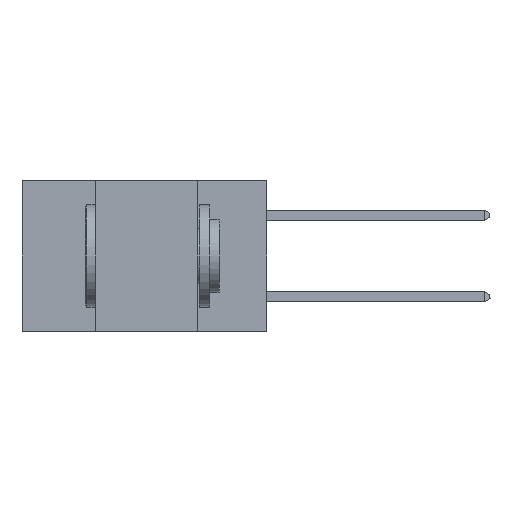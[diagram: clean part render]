
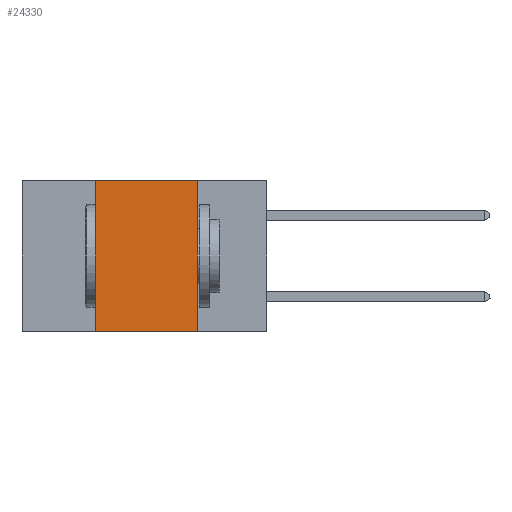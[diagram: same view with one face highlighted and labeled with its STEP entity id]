
A CAD part, left-side view. The second image highlights one B-rep face of the part: STEP entity #24330.
In plain terms, the highlighted planar face has unit normal (-1, 0, 0).
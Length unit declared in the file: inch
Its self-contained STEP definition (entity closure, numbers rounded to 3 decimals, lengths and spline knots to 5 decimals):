
#986 = DIRECTION ( 'NONE',  ( 0., -1., 0. ) ) ;
#1593 = ORIENTED_EDGE ( 'NONE', *, *, #7599, .F. ) ;
#2461 = LINE ( 'NONE', #20238, #40296 ) ;
#3059 = PLANE ( 'NONE',  #24854 ) ;
#5231 = EDGE_LOOP ( 'NONE', ( #1593, #37688, #17254, #7945 ) ) ;
#7599 = EDGE_CURVE ( 'NONE', #35448, #24059, #31156, .T. ) ;
#7945 = ORIENTED_EDGE ( 'NONE', *, *, #44711, .T. ) ;
#10619 = DIRECTION ( 'NONE',  ( 0., 0., -1. ) ) ;
#13319 = VERTEX_POINT ( 'NONE', #16702 ) ;
#15252 = EDGE_CURVE ( 'NONE', #38961, #35448, #2461, .T. ) ;
#16702 = CARTESIAN_POINT ( 'NONE',  ( 0., 0.42, -0.37 ) ) ;
#17254 = ORIENTED_EDGE ( 'NONE', *, *, #38157, .F. ) ;
#17668 = CARTESIAN_POINT ( 'NONE',  ( 0., 0.42, 0. ) ) ;
#20238 = CARTESIAN_POINT ( 'NONE',  ( 0., 0.6, 0. ) ) ;
#20948 = LINE ( 'NONE', #17668, #39075 ) ;
#21312 = CARTESIAN_POINT ( 'NONE',  ( 0., 0.17, 0. ) ) ;
#21463 = VECTOR ( 'NONE', #32284, 39.37008 ) ;
#22264 = LINE ( 'NONE', #44858, #40348 ) ;
#22502 = CARTESIAN_POINT ( 'NONE',  ( 0., 0.17, 0. ) ) ;
#24059 = VERTEX_POINT ( 'NONE', #45426 ) ;
#24330 = ADVANCED_FACE ( 'NONE', ( #41586 ), #3059, .F. ) ;
#24854 = AXIS2_PLACEMENT_3D ( 'NONE', #28909, #32529, #10619 ) ;
#28909 = CARTESIAN_POINT ( 'NONE',  ( 0., 0.6, 0. ) ) ;
#31156 = LINE ( 'NONE', #21312, #21463 ) ;
#32284 = DIRECTION ( 'NONE',  ( 0., 0., -1. ) ) ;
#32529 = DIRECTION ( 'NONE',  ( 1., 0., 0. ) ) ;
#33016 = CARTESIAN_POINT ( 'NONE',  ( 0., 0.42, 0. ) ) ;
#35448 = VERTEX_POINT ( 'NONE', #22502 ) ;
#37688 = ORIENTED_EDGE ( 'NONE', *, *, #15252, .F. ) ;
#38157 = EDGE_CURVE ( 'NONE', #13319, #38961, #20948, .T. ) ;
#38961 = VERTEX_POINT ( 'NONE', #33016 ) ;
#39075 = VECTOR ( 'NONE', #46593, 39.37008 ) ;
#40296 = VECTOR ( 'NONE', #41876, 39.37008 ) ;
#40348 = VECTOR ( 'NONE', #986, 39.37008 ) ;
#41586 = FACE_OUTER_BOUND ( 'NONE', #5231, .T. ) ;
#41876 = DIRECTION ( 'NONE',  ( 0., -1., 0. ) ) ;
#44711 = EDGE_CURVE ( 'NONE', #13319, #24059, #22264, .T. ) ;
#44858 = CARTESIAN_POINT ( 'NONE',  ( 0., 0.6, -0.37 ) ) ;
#45426 = CARTESIAN_POINT ( 'NONE',  ( 0., 0.17, -0.37 ) ) ;
#46593 = DIRECTION ( 'NONE',  ( 0., 0., 1. ) ) ;
